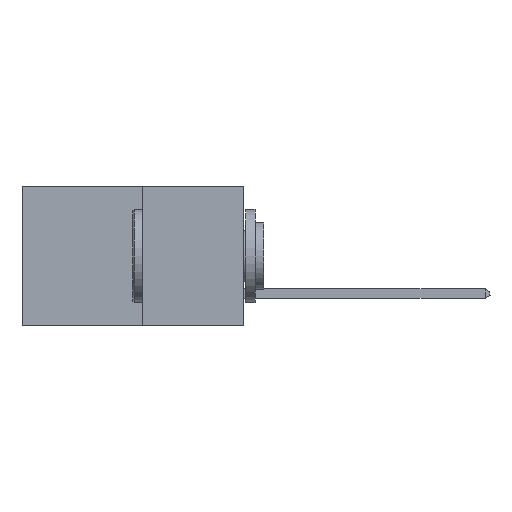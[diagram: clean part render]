
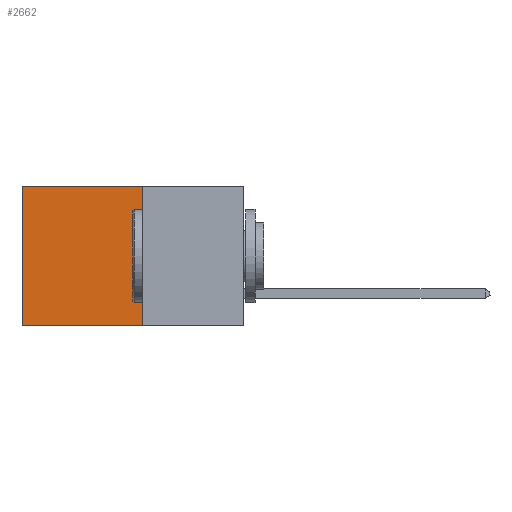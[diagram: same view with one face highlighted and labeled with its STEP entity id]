
A CAD part, left-side view. The second image highlights one B-rep face of the part: STEP entity #2662.
In plain terms, the highlighted planar face has unit normal (-1, 0, 0).
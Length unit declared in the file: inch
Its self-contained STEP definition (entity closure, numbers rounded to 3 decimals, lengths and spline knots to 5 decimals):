
#450 = DIRECTION ( 'NONE',  ( 0., 1., 0. ) ) ;
#1904 = AXIS2_PLACEMENT_3D ( 'NONE', #4482, #2634, #2557 ) ;
#2557 = DIRECTION ( 'NONE',  ( 0., 0., -1. ) ) ;
#2634 = DIRECTION ( 'NONE',  ( 1., 0., 0. ) ) ;
#2662 = ADVANCED_FACE ( 'NONE', ( #2821 ), #3421, .F. ) ;
#2731 = LINE ( 'NONE', #23998, #8891 ) ;
#2821 = FACE_OUTER_BOUND ( 'NONE', #9214, .T. ) ;
#3421 = PLANE ( 'NONE',  #1904 ) ;
#3454 = LINE ( 'NONE', #5072, #15769 ) ;
#4383 = CARTESIAN_POINT ( 'NONE',  ( 0.277, 0.27, -0.37 ) ) ;
#4482 = CARTESIAN_POINT ( 'NONE',  ( 0.277, 0.27, -0.37 ) ) ;
#5072 = CARTESIAN_POINT ( 'NONE',  ( 0.277, 0.27, 0. ) ) ;
#6207 = ORIENTED_EDGE ( 'NONE', *, *, #25971, .T. ) ;
#8891 = VECTOR ( 'NONE', #450, 39.37008 ) ;
#9214 = EDGE_LOOP ( 'NONE', ( #6207, #11921, #17241, #22328 ) ) ;
#10472 = LINE ( 'NONE', #19944, #17415 ) ;
#11921 = ORIENTED_EDGE ( 'NONE', *, *, #24551, .F. ) ;
#11979 = DIRECTION ( 'NONE',  ( 0., 0., -1. ) ) ;
#12364 = CARTESIAN_POINT ( 'NONE',  ( 0.277, 0.27, -0.37 ) ) ;
#14163 = CARTESIAN_POINT ( 'NONE',  ( 0.277, 0.59, -0.37 ) ) ;
#14297 = EDGE_CURVE ( 'NONE', #20911, #26492, #3454, .T. ) ;
#15769 = VECTOR ( 'NONE', #28678, 39.37008 ) ;
#17241 = ORIENTED_EDGE ( 'NONE', *, *, #20396, .F. ) ;
#17415 = VECTOR ( 'NONE', #11979, 39.37008 ) ;
#18774 = VERTEX_POINT ( 'NONE', #14163 ) ;
#19944 = CARTESIAN_POINT ( 'NONE',  ( 0.277, 0.59, -0.37 ) ) ;
#20396 = EDGE_CURVE ( 'NONE', #20911, #23657, #21360, .T. ) ;
#20531 = VECTOR ( 'NONE', #30614, 39.37008 ) ;
#20911 = VERTEX_POINT ( 'NONE', #22208 ) ;
#21360 = LINE ( 'NONE', #4383, #20531 ) ;
#22208 = CARTESIAN_POINT ( 'NONE',  ( 0.277, 0.27, 0. ) ) ;
#22328 = ORIENTED_EDGE ( 'NONE', *, *, #14297, .T. ) ;
#23657 = VERTEX_POINT ( 'NONE', #12364 ) ;
#23998 = CARTESIAN_POINT ( 'NONE',  ( 0.277, 0.27, -0.37 ) ) ;
#24551 = EDGE_CURVE ( 'NONE', #23657, #18774, #2731, .T. ) ;
#25971 = EDGE_CURVE ( 'NONE', #26492, #18774, #10472, .T. ) ;
#26492 = VERTEX_POINT ( 'NONE', #30009 ) ;
#28678 = DIRECTION ( 'NONE',  ( 0., 1., 0. ) ) ;
#30009 = CARTESIAN_POINT ( 'NONE',  ( 0.277, 0.59, 0. ) ) ;
#30614 = DIRECTION ( 'NONE',  ( 0., 0., -1. ) ) ;
